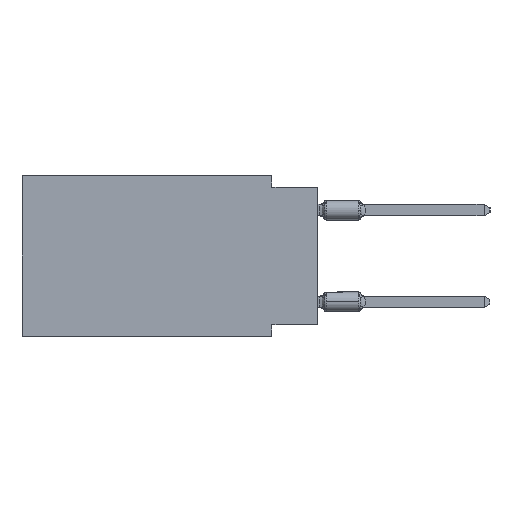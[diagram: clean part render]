
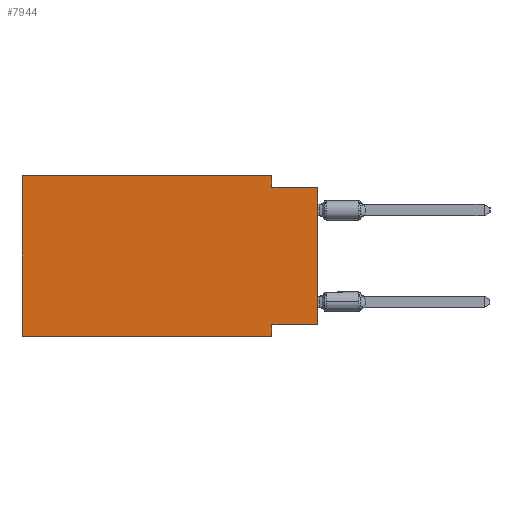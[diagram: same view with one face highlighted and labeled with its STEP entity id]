
A CAD part, left-side view. The second image highlights one B-rep face of the part: STEP entity #7944.
In plain terms, the highlighted planar face has unit normal (-1, 0, 0).
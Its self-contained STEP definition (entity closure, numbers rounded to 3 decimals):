
#262 = VECTOR ( 'NONE', #15841, 1000. ) ;
#447 = LINE ( 'NONE', #8563, #9230 ) ;
#636 = ORIENTED_EDGE ( 'NONE', *, *, #22600, .F. ) ;
#689 = VECTOR ( 'NONE', #19436, 1000. ) ;
#1231 = DIRECTION ( 'NONE',  ( 1., 0., 0. ) ) ;
#1424 = EDGE_CURVE ( 'NONE', #13954, #11553, #447, .T. ) ;
#1495 = EDGE_CURVE ( 'NONE', #9802, #13791, #5607, .T. ) ;
#1498 = CARTESIAN_POINT ( 'NONE',  ( 0., 16.383, 0. ) ) ;
#2126 = CARTESIAN_POINT ( 'NONE',  ( 0., 2.54, 0. ) ) ;
#2304 = EDGE_LOOP ( 'NONE', ( #13964, #8263, #636, #18200, #17719, #8139, #16263, #8427 ) ) ;
#3521 = LINE ( 'NONE', #9661, #22810 ) ;
#4208 = CARTESIAN_POINT ( 'NONE',  ( 0., 0., 0. ) ) ;
#4423 = CARTESIAN_POINT ( 'NONE',  ( 0., 2.54, -8.89 ) ) ;
#5208 = CARTESIAN_POINT ( 'NONE',  ( 0., 16.383, -8.89 ) ) ;
#5344 = DIRECTION ( 'NONE',  ( 0., 0., -1. ) ) ;
#5607 = LINE ( 'NONE', #9611, #689 ) ;
#6164 = CARTESIAN_POINT ( 'NONE',  ( 0., 2.54, 0. ) ) ;
#6419 = EDGE_CURVE ( 'NONE', #11134, #13990, #12278, .T. ) ;
#7292 = EDGE_CURVE ( 'NONE', #13087, #13791, #12573, .T. ) ;
#7938 = VERTEX_POINT ( 'NONE', #5208 ) ;
#7944 = ADVANCED_FACE ( 'NONE', ( #9609 ), #21416, .F. ) ;
#8139 = ORIENTED_EDGE ( 'NONE', *, *, #15287, .T. ) ;
#8213 = CARTESIAN_POINT ( 'NONE',  ( 0., 16.383, 0. ) ) ;
#8263 = ORIENTED_EDGE ( 'NONE', *, *, #1495, .F. ) ;
#8279 = CARTESIAN_POINT ( 'NONE',  ( 0., 2.54, -8.255 ) ) ;
#8427 = ORIENTED_EDGE ( 'NONE', *, *, #15408, .F. ) ;
#8563 = CARTESIAN_POINT ( 'NONE',  ( 0., 16.383, 0. ) ) ;
#9127 = DIRECTION ( 'NONE',  ( 0., -1., 0. ) ) ;
#9230 = VECTOR ( 'NONE', #19046, 1000. ) ;
#9400 = CARTESIAN_POINT ( 'NONE',  ( 0., 2.54, -0.635 ) ) ;
#9609 = FACE_OUTER_BOUND ( 'NONE', #2304, .T. ) ;
#9611 = CARTESIAN_POINT ( 'NONE',  ( 0., 0., -0.635 ) ) ;
#9661 = CARTESIAN_POINT ( 'NONE',  ( 0., 0., -8.255 ) ) ;
#9802 = VERTEX_POINT ( 'NONE', #9400 ) ;
#10153 = LINE ( 'NONE', #6164, #18539 ) ;
#11134 = VERTEX_POINT ( 'NONE', #8279 ) ;
#11278 = VECTOR ( 'NONE', #14304, 1000. ) ;
#11553 = VERTEX_POINT ( 'NONE', #2126 ) ;
#11725 = CARTESIAN_POINT ( 'NONE',  ( 0., 16.383, 0. ) ) ;
#12278 = LINE ( 'NONE', #4423, #12503 ) ;
#12503 = VECTOR ( 'NONE', #16008, 1000. ) ;
#12573 = LINE ( 'NONE', #4208, #11278 ) ;
#13087 = VERTEX_POINT ( 'NONE', #20174 ) ;
#13585 = LINE ( 'NONE', #1498, #262 ) ;
#13763 = EDGE_CURVE ( 'NONE', #7938, #13954, #13585, .T. ) ;
#13791 = VERTEX_POINT ( 'NONE', #26199 ) ;
#13908 = VECTOR ( 'NONE', #9127, 1000. ) ;
#13954 = VERTEX_POINT ( 'NONE', #8213 ) ;
#13964 = ORIENTED_EDGE ( 'NONE', *, *, #7292, .T. ) ;
#13990 = VERTEX_POINT ( 'NONE', #20935 ) ;
#14252 = DIRECTION ( 'NONE',  ( 0., 0., -1. ) ) ;
#14304 = DIRECTION ( 'NONE',  ( 0., 0., 1. ) ) ;
#15097 = LINE ( 'NONE', #23059, #13908 ) ;
#15287 = EDGE_CURVE ( 'NONE', #7938, #13990, #15097, .T. ) ;
#15408 = EDGE_CURVE ( 'NONE', #13087, #11134, #3521, .T. ) ;
#15841 = DIRECTION ( 'NONE',  ( 0., 0., 1. ) ) ;
#16008 = DIRECTION ( 'NONE',  ( 0., 0., -1. ) ) ;
#16263 = ORIENTED_EDGE ( 'NONE', *, *, #6419, .F. ) ;
#17719 = ORIENTED_EDGE ( 'NONE', *, *, #13763, .F. ) ;
#18200 = ORIENTED_EDGE ( 'NONE', *, *, #1424, .F. ) ;
#18539 = VECTOR ( 'NONE', #14252, 1000. ) ;
#19046 = DIRECTION ( 'NONE',  ( 0., -1., 0. ) ) ;
#19436 = DIRECTION ( 'NONE',  ( 0., -1., 0. ) ) ;
#19873 = DIRECTION ( 'NONE',  ( 0., 1., 0. ) ) ;
#20174 = CARTESIAN_POINT ( 'NONE',  ( 0., 0., -8.255 ) ) ;
#20606 = AXIS2_PLACEMENT_3D ( 'NONE', #11725, #1231, #5344 ) ;
#20935 = CARTESIAN_POINT ( 'NONE',  ( 0., 2.54, -8.89 ) ) ;
#21416 = PLANE ( 'NONE',  #20606 ) ;
#22600 = EDGE_CURVE ( 'NONE', #11553, #9802, #10153, .T. ) ;
#22810 = VECTOR ( 'NONE', #19873, 1000. ) ;
#23059 = CARTESIAN_POINT ( 'NONE',  ( 0., 16.383, -8.89 ) ) ;
#26199 = CARTESIAN_POINT ( 'NONE',  ( 0., 0., -0.635 ) ) ;
